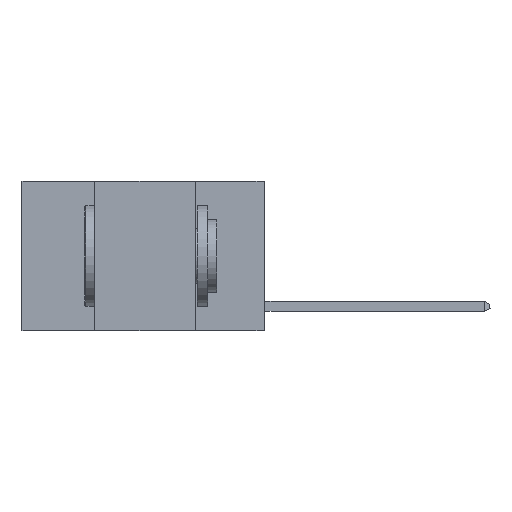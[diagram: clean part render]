
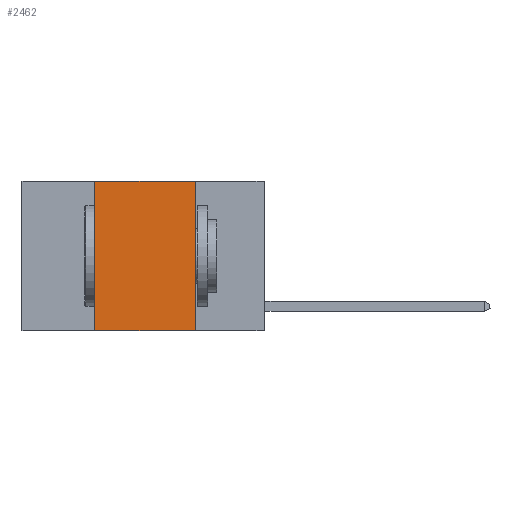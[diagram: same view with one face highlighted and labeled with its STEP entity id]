
A CAD part, left-side view. The second image highlights one B-rep face of the part: STEP entity #2462.
In plain terms, the highlighted planar face has unit normal (-1, 0, 0).
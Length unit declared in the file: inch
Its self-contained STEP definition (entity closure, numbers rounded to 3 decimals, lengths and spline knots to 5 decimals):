
#3 = FACE_OUTER_BOUND ( 'NONE', #11905, .T. ) ;
#73 = CARTESIAN_POINT ( 'NONE',  ( 0., 0.6, 0. ) ) ;
#107 = EDGE_CURVE ( 'NONE', #10288, #1008, #3676, .T. ) ;
#1008 = VERTEX_POINT ( 'NONE', #3003 ) ;
#2444 = EDGE_CURVE ( 'NONE', #10288, #2507, #3066, .T. ) ;
#2462 = ADVANCED_FACE ( 'NONE', ( #3 ), #8446, .F. ) ;
#2507 = VERTEX_POINT ( 'NONE', #9613 ) ;
#2744 = VECTOR ( 'NONE', #10084, 39.37008 ) ;
#2789 = CARTESIAN_POINT ( 'NONE',  ( 0., 0.17, 0. ) ) ;
#2895 = VERTEX_POINT ( 'NONE', #12785 ) ;
#3003 = CARTESIAN_POINT ( 'NONE',  ( 0., 0.42, 0. ) ) ;
#3009 = DIRECTION ( 'NONE',  ( 0., -1., 0. ) ) ;
#3066 = LINE ( 'NONE', #8525, #8059 ) ;
#3482 = CARTESIAN_POINT ( 'NONE',  ( 0., 0.42, -0.37 ) ) ;
#3662 = EDGE_CURVE ( 'NONE', #1008, #2895, #13386, .T. ) ;
#3676 = LINE ( 'NONE', #6059, #2744 ) ;
#4282 = ORIENTED_EDGE ( 'NONE', *, *, #3662, .F. ) ;
#4534 = ORIENTED_EDGE ( 'NONE', *, *, #107, .F. ) ;
#6059 = CARTESIAN_POINT ( 'NONE',  ( 0., 0.42, 0. ) ) ;
#7168 = AXIS2_PLACEMENT_3D ( 'NONE', #73, #11756, #12822 ) ;
#8059 = VECTOR ( 'NONE', #10644, 39.37008 ) ;
#8446 = PLANE ( 'NONE',  #7168 ) ;
#8525 = CARTESIAN_POINT ( 'NONE',  ( 0., 0.6, -0.37 ) ) ;
#9613 = CARTESIAN_POINT ( 'NONE',  ( 0., 0.17, -0.37 ) ) ;
#9955 = DIRECTION ( 'NONE',  ( 0., 0., -1. ) ) ;
#10084 = DIRECTION ( 'NONE',  ( 0., 0., 1. ) ) ;
#10288 = VERTEX_POINT ( 'NONE', #3482 ) ;
#10401 = EDGE_CURVE ( 'NONE', #2895, #2507, #12170, .T. ) ;
#10644 = DIRECTION ( 'NONE',  ( 0., -1., 0. ) ) ;
#11283 = VECTOR ( 'NONE', #9955, 39.37008 ) ;
#11445 = ORIENTED_EDGE ( 'NONE', *, *, #2444, .T. ) ;
#11756 = DIRECTION ( 'NONE',  ( 1., 0., 0. ) ) ;
#11905 = EDGE_LOOP ( 'NONE', ( #13687, #4282, #4534, #11445 ) ) ;
#12170 = LINE ( 'NONE', #2789, #11283 ) ;
#12785 = CARTESIAN_POINT ( 'NONE',  ( 0., 0.17, 0. ) ) ;
#12822 = DIRECTION ( 'NONE',  ( 0., 0., -1. ) ) ;
#13085 = VECTOR ( 'NONE', #3009, 39.37008 ) ;
#13386 = LINE ( 'NONE', #13589, #13085 ) ;
#13589 = CARTESIAN_POINT ( 'NONE',  ( 0., 0.6, 0. ) ) ;
#13687 = ORIENTED_EDGE ( 'NONE', *, *, #10401, .F. ) ;
